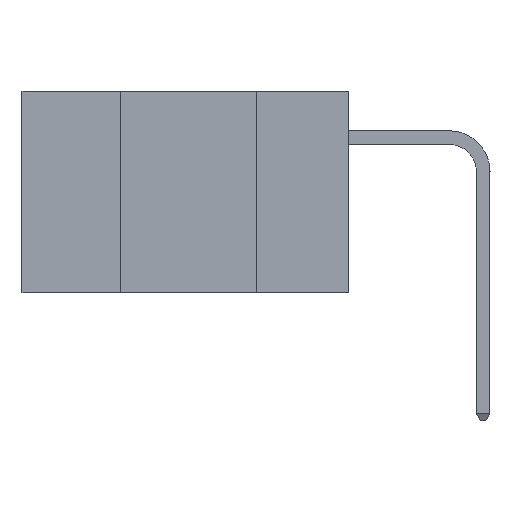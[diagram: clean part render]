
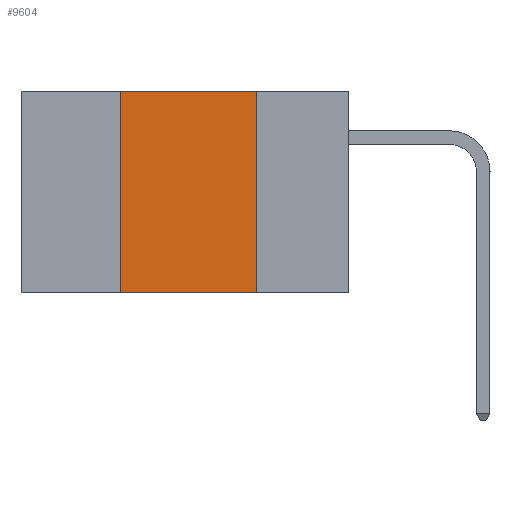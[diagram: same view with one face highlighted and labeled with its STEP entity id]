
A CAD part, left-side view. The second image highlights one B-rep face of the part: STEP entity #9604.
In plain terms, the highlighted planar face has unit normal (-1, 0, 0).
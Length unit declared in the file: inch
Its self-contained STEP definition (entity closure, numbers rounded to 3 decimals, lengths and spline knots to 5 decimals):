
#44 = ORIENTED_EDGE ( 'NONE', *, *, #1881, .T. ) ;
#961 = EDGE_LOOP ( 'NONE', ( #1217, #6582, #4915, #44 ) ) ;
#1217 = ORIENTED_EDGE ( 'NONE', *, *, #16575, .F. ) ;
#1369 = EDGE_CURVE ( 'NONE', #2829, #9024, #4632, .T. ) ;
#1689 = CARTESIAN_POINT ( 'NONE',  ( 0., 0.17, -0.37 ) ) ;
#1881 = EDGE_CURVE ( 'NONE', #10999, #10158, #7356, .T. ) ;
#2242 = EDGE_CURVE ( 'NONE', #10999, #2829, #16674, .T. ) ;
#2389 = CARTESIAN_POINT ( 'NONE',  ( 0., 0.42, 0. ) ) ;
#2829 = VERTEX_POINT ( 'NONE', #16204 ) ;
#3652 = CARTESIAN_POINT ( 'NONE',  ( 0., 0.6, -0.37 ) ) ;
#4560 = DIRECTION ( 'NONE',  ( 0., -1., 0. ) ) ;
#4632 = LINE ( 'NONE', #8188, #8223 ) ;
#4715 = CARTESIAN_POINT ( 'NONE',  ( 0., 0.17, 0. ) ) ;
#4915 = ORIENTED_EDGE ( 'NONE', *, *, #2242, .F. ) ;
#5923 = PLANE ( 'NONE',  #11529 ) ;
#6582 = ORIENTED_EDGE ( 'NONE', *, *, #1369, .F. ) ;
#7282 = DIRECTION ( 'NONE',  ( 1., 0., 0. ) ) ;
#7356 = LINE ( 'NONE', #3652, #13845 ) ;
#7742 = CARTESIAN_POINT ( 'NONE',  ( 0., 0.42, -0.37 ) ) ;
#8188 = CARTESIAN_POINT ( 'NONE',  ( 0., 0.6, 0. ) ) ;
#8223 = VECTOR ( 'NONE', #4560, 39.37008 ) ;
#9024 = VERTEX_POINT ( 'NONE', #4715 ) ;
#9347 = FACE_OUTER_BOUND ( 'NONE', #961, .T. ) ;
#9373 = DIRECTION ( 'NONE',  ( 0., -1., 0. ) ) ;
#9604 = ADVANCED_FACE ( 'NONE', ( #9347 ), #5923, .F. ) ;
#10158 = VERTEX_POINT ( 'NONE', #1689 ) ;
#10999 = VERTEX_POINT ( 'NONE', #7742 ) ;
#11103 = VECTOR ( 'NONE', #13948, 39.37008 ) ;
#11529 = AXIS2_PLACEMENT_3D ( 'NONE', #15003, #7282, #16278 ) ;
#13845 = VECTOR ( 'NONE', #9373, 39.37008 ) ;
#13948 = DIRECTION ( 'NONE',  ( 0., 0., -1. ) ) ;
#14479 = LINE ( 'NONE', #15184, #11103 ) ;
#15003 = CARTESIAN_POINT ( 'NONE',  ( 0., 0.6, 0. ) ) ;
#15184 = CARTESIAN_POINT ( 'NONE',  ( 0., 0.17, 0. ) ) ;
#16204 = CARTESIAN_POINT ( 'NONE',  ( 0., 0.42, 0. ) ) ;
#16278 = DIRECTION ( 'NONE',  ( 0., 0., -1. ) ) ;
#16286 = VECTOR ( 'NONE', #16868, 39.37008 ) ;
#16575 = EDGE_CURVE ( 'NONE', #9024, #10158, #14479, .T. ) ;
#16674 = LINE ( 'NONE', #2389, #16286 ) ;
#16868 = DIRECTION ( 'NONE',  ( 0., 0., 1. ) ) ;
